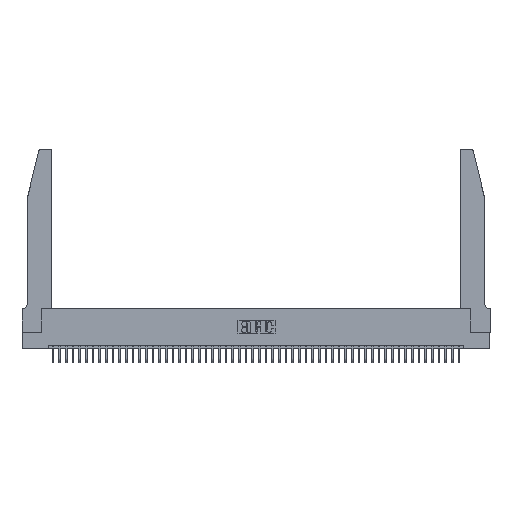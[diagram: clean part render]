
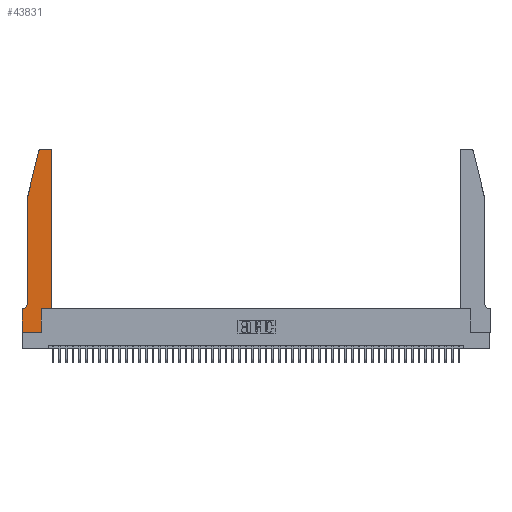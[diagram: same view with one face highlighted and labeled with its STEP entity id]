
A CAD part, top view. The second image highlights one B-rep face of the part: STEP entity #43831.
In plain terms, the highlighted planar face has unit normal (0, 0, 1).
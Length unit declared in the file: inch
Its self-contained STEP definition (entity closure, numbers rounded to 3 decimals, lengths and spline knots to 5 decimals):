
#493 = ORIENTED_EDGE ( 'NONE', *, *, #47286, .T. ) ;
#583 = LINE ( 'NONE', #35888, #21140 ) ;
#661 = CARTESIAN_POINT ( 'NONE',  ( 0., 0.35, 0.37 ) ) ;
#799 = DIRECTION ( 'NONE',  ( -1., 0., 0. ) ) ;
#1116 = VERTEX_POINT ( 'NONE', #15434 ) ;
#1206 = VERTEX_POINT ( 'NONE', #8477 ) ;
#1617 = VERTEX_POINT ( 'NONE', #19025 ) ;
#2571 = CARTESIAN_POINT ( 'NONE',  ( 0.2605, 2.75, 0.37 ) ) ;
#4819 = DIRECTION ( 'NONE',  ( 0., 0., 1. ) ) ;
#4912 = EDGE_CURVE ( 'NONE', #1206, #41875, #583, .T. ) ;
#5341 = VECTOR ( 'NONE', #36864, 39.37008 ) ;
#5791 = VECTOR ( 'NONE', #28217, 39.37008 ) ;
#5956 = ORIENTED_EDGE ( 'NONE', *, *, #14545, .T. ) ;
#7719 = VERTEX_POINT ( 'NONE', #38992 ) ;
#8477 = CARTESIAN_POINT ( 'NONE',  ( 0.2865, 0., 0.37 ) ) ;
#8701 = CARTESIAN_POINT ( 'NONE',  ( 0., 0., 0.37 ) ) ;
#9003 = VERTEX_POINT ( 'NONE', #11286 ) ;
#11286 = CARTESIAN_POINT ( 'NONE',  ( 0., 0., 0.37 ) ) ;
#11495 = CARTESIAN_POINT ( 'NONE',  ( 0.4205, 2.72, 0.37 ) ) ;
#11603 = DIRECTION ( 'NONE',  ( 0., 1., 0. ) ) ;
#12259 = ORIENTED_EDGE ( 'NONE', *, *, #17273, .T. ) ;
#12578 = FACE_OUTER_BOUND ( 'NONE', #21407, .T. ) ;
#12818 = LINE ( 'NONE', #51038, #45010 ) ;
#14010 = DIRECTION ( 'NONE',  ( 1., 0., 0. ) ) ;
#14177 = DIRECTION ( 'NONE',  ( 0., 0., 1. ) ) ;
#14545 = EDGE_CURVE ( 'NONE', #24516, #39413, #31912, .T. ) ;
#14559 = ORIENTED_EDGE ( 'NONE', *, *, #25042, .T. ) ;
#14756 = DIRECTION ( 'NONE',  ( -1., 0., 0. ) ) ;
#15342 = DIRECTION ( 'NONE',  ( -1., 0., 0. ) ) ;
#15434 = CARTESIAN_POINT ( 'NONE',  ( 0.284, 2.75, 0.37 ) ) ;
#15603 = DIRECTION ( 'NONE',  ( 1., 0., 0. ) ) ;
#16333 = ORIENTED_EDGE ( 'NONE', *, *, #30918, .T. ) ;
#16791 = AXIS2_PLACEMENT_3D ( 'NONE', #11495, #39782, #15603 ) ;
#17273 = EDGE_CURVE ( 'NONE', #20716, #27167, #34875, .T. ) ;
#17499 = CARTESIAN_POINT ( 'NONE',  ( 0.4505, 2.72, 0.37 ) ) ;
#19025 = CARTESIAN_POINT ( 'NONE',  ( 0.0055, 0.35, 0.37 ) ) ;
#19968 = EDGE_CURVE ( 'NONE', #28107, #24516, #12818, .T. ) ;
#20716 = VERTEX_POINT ( 'NONE', #40820 ) ;
#21140 = VECTOR ( 'NONE', #11603, 39.37008 ) ;
#21184 = VECTOR ( 'NONE', #14010, 39.37008 ) ;
#21407 = EDGE_LOOP ( 'NONE', ( #32026, #49848, #14559, #12259, #25863, #28196, #16333, #23439, #33352, #493, #48405, #5956 ) ) ;
#21467 = EDGE_CURVE ( 'NONE', #27167, #1617, #37347, .T. ) ;
#22927 = VECTOR ( 'NONE', #33237, 39.37008 ) ;
#23439 = ORIENTED_EDGE ( 'NONE', *, *, #47584, .T. ) ;
#23992 = VECTOR ( 'NONE', #28989, 39.37008 ) ;
#24249 = DIRECTION ( 'NONE',  ( 0., 1., 0. ) ) ;
#24516 = VERTEX_POINT ( 'NONE', #17499 ) ;
#24747 = CARTESIAN_POINT ( 'NONE',  ( 0.0755, 2., 0.37 ) ) ;
#25042 = EDGE_CURVE ( 'NONE', #7719, #20716, #38965, .T. ) ;
#25185 = CARTESIAN_POINT ( 'NONE',  ( 0.0755, 2., 0.37 ) ) ;
#25207 = PLANE ( 'NONE',  #31503 ) ;
#25337 = DIRECTION ( 'NONE',  ( 0., 0., -1. ) ) ;
#25863 = ORIENTED_EDGE ( 'NONE', *, *, #21467, .T. ) ;
#27167 = VERTEX_POINT ( 'NONE', #43231 ) ;
#27757 = EDGE_CURVE ( 'NONE', #1617, #28053, #44917, .T. ) ;
#27801 = CARTESIAN_POINT ( 'NONE',  ( 0.2865, 0.35, 0.37 ) ) ;
#28053 = VERTEX_POINT ( 'NONE', #45238 ) ;
#28107 = VERTEX_POINT ( 'NONE', #37551 ) ;
#28196 = ORIENTED_EDGE ( 'NONE', *, *, #27757, .T. ) ;
#28217 = DIRECTION ( 'NONE',  ( 1., 0., 0. ) ) ;
#28431 = LINE ( 'NONE', #2571, #39074 ) ;
#28989 = DIRECTION ( 'NONE',  ( 0., -1., 0. ) ) ;
#29307 = CIRCLE ( 'NONE', #43641, 0.03 ) ;
#30918 = EDGE_CURVE ( 'NONE', #28053, #9003, #34692, .T. ) ;
#31503 = AXIS2_PLACEMENT_3D ( 'NONE', #661, #4819, #33251 ) ;
#31889 = LINE ( 'NONE', #38208, #21184 ) ;
#31912 = CIRCLE ( 'NONE', #16791, 0.03 ) ;
#32026 = ORIENTED_EDGE ( 'NONE', *, *, #40420, .T. ) ;
#32066 = CARTESIAN_POINT ( 'NONE',  ( 0.4205, 2.75, 0.37 ) ) ;
#33237 = DIRECTION ( 'NONE',  ( 0., -1., 0. ) ) ;
#33251 = DIRECTION ( 'NONE',  ( 1., 0., 0. ) ) ;
#33352 = ORIENTED_EDGE ( 'NONE', *, *, #4912, .T. ) ;
#34692 = LINE ( 'NONE', #8701, #23992 ) ;
#34875 = LINE ( 'NONE', #25185, #22927 ) ;
#35524 = CARTESIAN_POINT ( 'NONE',  ( 0.0755, 0.35, 0.37 ) ) ;
#35888 = CARTESIAN_POINT ( 'NONE',  ( 0.2865, 0.35, 0.37 ) ) ;
#36864 = DIRECTION ( 'NONE',  ( -0.239, -0.971, 0. ) ) ;
#37347 = CIRCLE ( 'NONE', #52352, 0.07 ) ;
#37551 = CARTESIAN_POINT ( 'NONE',  ( 0.4505, 0.35, 0.37 ) ) ;
#38127 = LINE ( 'NONE', #44109, #5791 ) ;
#38208 = CARTESIAN_POINT ( 'NONE',  ( 0.4505, 0.35, 0.37 ) ) ;
#38379 = CARTESIAN_POINT ( 'NONE',  ( 0.284, 2.72, 0.37 ) ) ;
#38965 = LINE ( 'NONE', #24747, #5341 ) ;
#38992 = CARTESIAN_POINT ( 'NONE',  ( 0.25487, 2.72718, 0.37 ) ) ;
#39074 = VECTOR ( 'NONE', #14756, 39.37008 ) ;
#39413 = VERTEX_POINT ( 'NONE', #32066 ) ;
#39782 = DIRECTION ( 'NONE',  ( 0., 0., 1. ) ) ;
#40420 = EDGE_CURVE ( 'NONE', #39413, #1116, #28431, .T. ) ;
#40820 = CARTESIAN_POINT ( 'NONE',  ( 0.0755, 2., 0.37 ) ) ;
#41875 = VERTEX_POINT ( 'NONE', #27801 ) ;
#42389 = DIRECTION ( 'NONE',  ( 1., 0., 0. ) ) ;
#43231 = CARTESIAN_POINT ( 'NONE',  ( 0.0755, 0.42, 0.37 ) ) ;
#43641 = AXIS2_PLACEMENT_3D ( 'NONE', #38379, #14177, #42389 ) ;
#43672 = VECTOR ( 'NONE', #15342, 39.37008 ) ;
#43831 = ADVANCED_FACE ( 'NONE', ( #12578 ), #25207, .T. ) ;
#44109 = CARTESIAN_POINT ( 'NONE',  ( 0., 0., 0.37 ) ) ;
#44917 = LINE ( 'NONE', #35524, #43672 ) ;
#45010 = VECTOR ( 'NONE', #24249, 39.37008 ) ;
#45238 = CARTESIAN_POINT ( 'NONE',  ( 0., 0.35, 0.37 ) ) ;
#47286 = EDGE_CURVE ( 'NONE', #41875, #28107, #31889, .T. ) ;
#47584 = EDGE_CURVE ( 'NONE', #9003, #1206, #38127, .T. ) ;
#48405 = ORIENTED_EDGE ( 'NONE', *, *, #19968, .T. ) ;
#49283 = CARTESIAN_POINT ( 'NONE',  ( 0.0055, 0.42, 0.37 ) ) ;
#49848 = ORIENTED_EDGE ( 'NONE', *, *, #51694, .T. ) ;
#51038 = CARTESIAN_POINT ( 'NONE',  ( 0.4505, 0.35, 0.37 ) ) ;
#51694 = EDGE_CURVE ( 'NONE', #1116, #7719, #29307, .T. ) ;
#52352 = AXIS2_PLACEMENT_3D ( 'NONE', #49283, #25337, #799 ) ;
